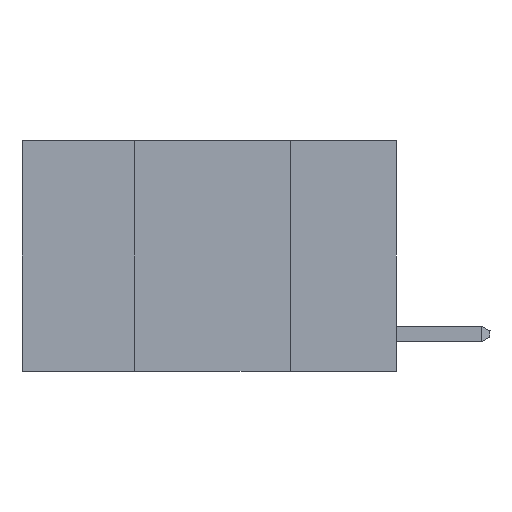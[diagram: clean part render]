
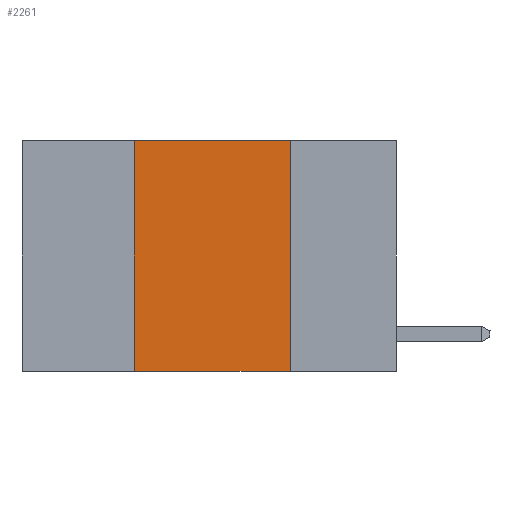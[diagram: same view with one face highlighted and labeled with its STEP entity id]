
A CAD part, left-side view. The second image highlights one B-rep face of the part: STEP entity #2261.
In plain terms, the highlighted planar face has unit normal (-1, 0, 0).
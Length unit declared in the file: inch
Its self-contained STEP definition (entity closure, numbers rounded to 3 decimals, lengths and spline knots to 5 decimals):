
#384 = LINE ( 'NONE', #14480, #17072 ) ;
#486 = VECTOR ( 'NONE', #16360, 39.37008 ) ;
#880 = AXIS2_PLACEMENT_3D ( 'NONE', #19487, #14757, #11656 ) ;
#965 = CARTESIAN_POINT ( 'NONE',  ( 0., 0.6, 0. ) ) ;
#1966 = EDGE_CURVE ( 'NONE', #2640, #10079, #5417, .T. ) ;
#2261 = ADVANCED_FACE ( 'NONE', ( #6823 ), #3918, .F. ) ;
#2640 = VERTEX_POINT ( 'NONE', #7737 ) ;
#3918 = PLANE ( 'NONE',  #880 ) ;
#4239 = DIRECTION ( 'NONE',  ( 0., -1., 0. ) ) ;
#5184 = CARTESIAN_POINT ( 'NONE',  ( 0., 0.17, -0.37 ) ) ;
#5320 = VERTEX_POINT ( 'NONE', #5184 ) ;
#5335 = VECTOR ( 'NONE', #11704, 39.37008 ) ;
#5417 = LINE ( 'NONE', #15013, #5335 ) ;
#5505 = ORIENTED_EDGE ( 'NONE', *, *, #9106, .T. ) ;
#6348 = ORIENTED_EDGE ( 'NONE', *, *, #15795, .F. ) ;
#6354 = ORIENTED_EDGE ( 'NONE', *, *, #15593, .F. ) ;
#6823 = FACE_OUTER_BOUND ( 'NONE', #8660, .T. ) ;
#7177 = LINE ( 'NONE', #13443, #486 ) ;
#7264 = VECTOR ( 'NONE', #4239, 39.37008 ) ;
#7629 = CARTESIAN_POINT ( 'NONE',  ( 0., 0.42, 0. ) ) ;
#7737 = CARTESIAN_POINT ( 'NONE',  ( 0., 0.42, -0.37 ) ) ;
#8660 = EDGE_LOOP ( 'NONE', ( #6354, #6348, #17993, #5505 ) ) ;
#9106 = EDGE_CURVE ( 'NONE', #2640, #5320, #7177, .T. ) ;
#9171 = VERTEX_POINT ( 'NONE', #9204 ) ;
#9204 = CARTESIAN_POINT ( 'NONE',  ( 0., 0.17, 0. ) ) ;
#10079 = VERTEX_POINT ( 'NONE', #7629 ) ;
#11656 = DIRECTION ( 'NONE',  ( 0., 0., -1. ) ) ;
#11704 = DIRECTION ( 'NONE',  ( 0., 0., 1. ) ) ;
#13443 = CARTESIAN_POINT ( 'NONE',  ( 0., 0.6, -0.37 ) ) ;
#14293 = DIRECTION ( 'NONE',  ( 0., 0., -1. ) ) ;
#14480 = CARTESIAN_POINT ( 'NONE',  ( 0., 0.17, 0. ) ) ;
#14757 = DIRECTION ( 'NONE',  ( 1., 0., 0. ) ) ;
#15013 = CARTESIAN_POINT ( 'NONE',  ( 0., 0.42, 0. ) ) ;
#15593 = EDGE_CURVE ( 'NONE', #9171, #5320, #384, .T. ) ;
#15795 = EDGE_CURVE ( 'NONE', #10079, #9171, #16725, .T. ) ;
#16360 = DIRECTION ( 'NONE',  ( 0., -1., 0. ) ) ;
#16725 = LINE ( 'NONE', #965, #7264 ) ;
#17072 = VECTOR ( 'NONE', #14293, 39.37008 ) ;
#17993 = ORIENTED_EDGE ( 'NONE', *, *, #1966, .F. ) ;
#19487 = CARTESIAN_POINT ( 'NONE',  ( 0., 0.6, 0. ) ) ;
